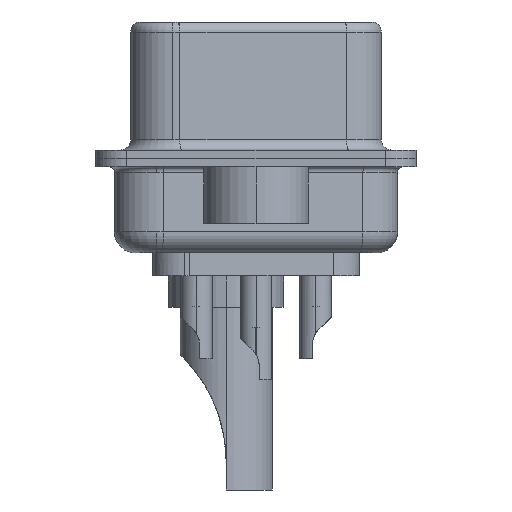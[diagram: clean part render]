
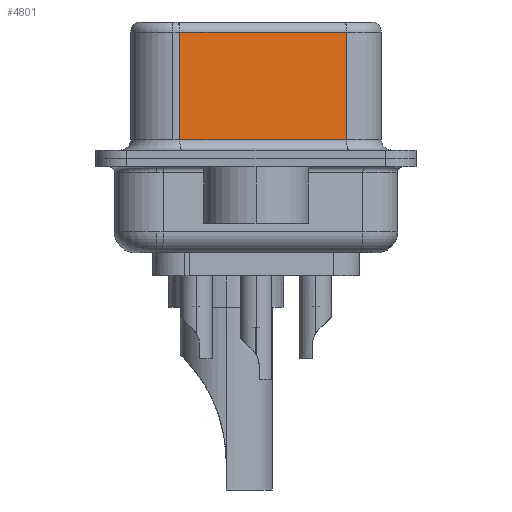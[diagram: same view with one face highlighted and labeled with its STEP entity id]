
A CAD part, left-side view. The second image highlights one B-rep face of the part: STEP entity #4801.
In plain terms, the highlighted planar face has unit normal (-0.985, -0.174, 0).
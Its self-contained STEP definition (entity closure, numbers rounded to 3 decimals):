
#831 = CARTESIAN_POINT ( 'NONE',  ( 5.132, -4.322, 6.02 ) ) ;
#1523 = VERTEX_POINT ( 'NONE', #24669 ) ;
#2089 = EDGE_LOOP ( 'NONE', ( #19975, #4640, #29231, #15823 ) ) ;
#2588 = EDGE_CURVE ( 'NONE', #1523, #12244, #2885, .T. ) ;
#2819 = VECTOR ( 'NONE', #12254, 1000. ) ;
#2885 = LINE ( 'NONE', #13077, #17316 ) ;
#4640 = ORIENTED_EDGE ( 'NONE', *, *, #17243, .T. ) ;
#4716 = DIRECTION ( 'NONE',  ( 0., 0., -1. ) ) ;
#4801 = ADVANCED_FACE ( 'NONE', ( #27263 ), #19443, .F. ) ;
#6860 = CARTESIAN_POINT ( 'NONE',  ( 3.73, 3.628, 6.52 ) ) ;
#8851 = VECTOR ( 'NONE', #15947, 1000. ) ;
#8980 = LINE ( 'NONE', #831, #2819 ) ;
#9860 = VECTOR ( 'NONE', #4716, 1000. ) ;
#10211 = DIRECTION ( 'NONE',  ( 0.985, 0.174, 0. ) ) ;
#11302 = CARTESIAN_POINT ( 'NONE',  ( 5.132, -4.322, 0.9 ) ) ;
#12244 = VERTEX_POINT ( 'NONE', #14965 ) ;
#12254 = DIRECTION ( 'NONE',  ( -0.174, 0.985, 0. ) ) ;
#13077 = CARTESIAN_POINT ( 'NONE',  ( 5.132, -4.322, 6.52 ) ) ;
#13878 = LINE ( 'NONE', #11302, #8851 ) ;
#14965 = CARTESIAN_POINT ( 'NONE',  ( 5.132, -4.322, 0.9 ) ) ;
#15823 = ORIENTED_EDGE ( 'NONE', *, *, #21740, .T. ) ;
#15947 = DIRECTION ( 'NONE',  ( 0.174, -0.985, 0. ) ) ;
#16880 = CARTESIAN_POINT ( 'NONE',  ( 3.73, 3.628, 0.9 ) ) ;
#17243 = EDGE_CURVE ( 'NONE', #1523, #23076, #8980, .T. ) ;
#17316 = VECTOR ( 'NONE', #22310, 1000. ) ;
#17654 = VERTEX_POINT ( 'NONE', #16880 ) ;
#19443 = PLANE ( 'NONE',  #24346 ) ;
#19975 = ORIENTED_EDGE ( 'NONE', *, *, #2588, .F. ) ;
#21740 = EDGE_CURVE ( 'NONE', #17654, #12244, #13878, .T. ) ;
#22310 = DIRECTION ( 'NONE',  ( 0., 0., -1. ) ) ;
#23076 = VERTEX_POINT ( 'NONE', #25393 ) ;
#24206 = EDGE_CURVE ( 'NONE', #23076, #17654, #27828, .T. ) ;
#24272 = CARTESIAN_POINT ( 'NONE',  ( 5.132, -4.322, 6.52 ) ) ;
#24346 = AXIS2_PLACEMENT_3D ( 'NONE', #24272, #10211, #28687 ) ;
#24669 = CARTESIAN_POINT ( 'NONE',  ( 5.132, -4.322, 6.02 ) ) ;
#25393 = CARTESIAN_POINT ( 'NONE',  ( 3.73, 3.628, 6.02 ) ) ;
#27263 = FACE_OUTER_BOUND ( 'NONE', #2089, .T. ) ;
#27828 = LINE ( 'NONE', #6860, #9860 ) ;
#28687 = DIRECTION ( 'NONE',  ( -0.174, 0.985, 0. ) ) ;
#29231 = ORIENTED_EDGE ( 'NONE', *, *, #24206, .T. ) ;
